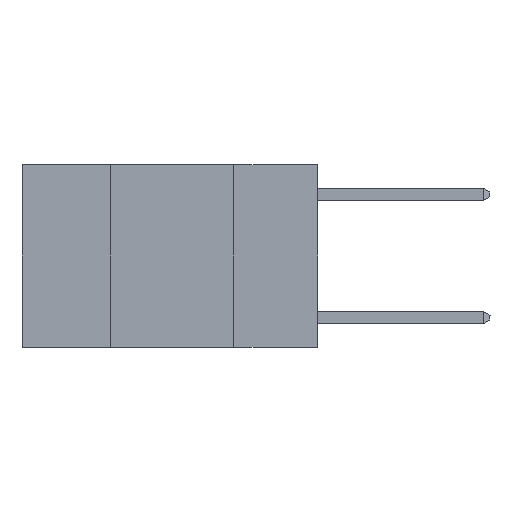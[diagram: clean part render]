
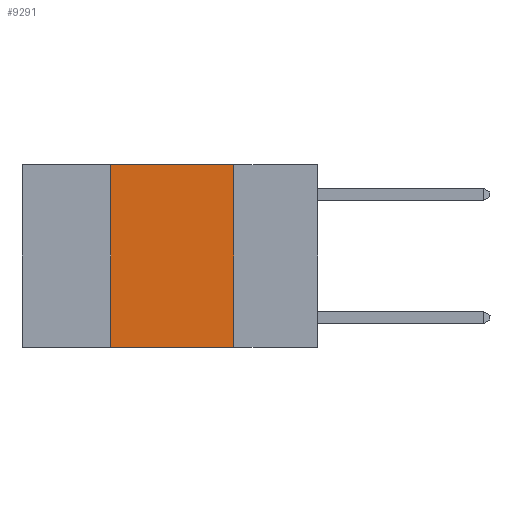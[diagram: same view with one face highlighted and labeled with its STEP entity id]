
A CAD part, left-side view. The second image highlights one B-rep face of the part: STEP entity #9291.
In plain terms, the highlighted planar face has unit normal (-1, 0, 0).
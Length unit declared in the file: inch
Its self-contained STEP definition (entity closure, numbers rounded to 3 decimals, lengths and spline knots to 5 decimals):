
#152 = EDGE_CURVE ( 'NONE', #15434, #3677, #10965, .T. ) ;
#878 = CARTESIAN_POINT ( 'NONE',  ( 0., 0.17, -0.37 ) ) ;
#952 = DIRECTION ( 'NONE',  ( 0., 0., 1. ) ) ;
#1786 = VERTEX_POINT ( 'NONE', #878 ) ;
#1881 = ORIENTED_EDGE ( 'NONE', *, *, #3883, .F. ) ;
#2121 = CARTESIAN_POINT ( 'NONE',  ( 0., 0.42, 0. ) ) ;
#2293 = LINE ( 'NONE', #8303, #11651 ) ;
#2453 = CARTESIAN_POINT ( 'NONE',  ( 0., 0.17, 0. ) ) ;
#2955 = PLANE ( 'NONE',  #13472 ) ;
#3048 = EDGE_CURVE ( 'NONE', #9590, #15434, #2293, .T. ) ;
#3677 = VERTEX_POINT ( 'NONE', #15465 ) ;
#3883 = EDGE_CURVE ( 'NONE', #3677, #1786, #9925, .T. ) ;
#4210 = DIRECTION ( 'NONE',  ( 0., 0., -1. ) ) ;
#4940 = LINE ( 'NONE', #14608, #14290 ) ;
#5136 = ORIENTED_EDGE ( 'NONE', *, *, #152, .F. ) ;
#6676 = VECTOR ( 'NONE', #14672, 39.37008 ) ;
#7719 = EDGE_LOOP ( 'NONE', ( #1881, #5136, #11629, #8777 ) ) ;
#7736 = VECTOR ( 'NONE', #9434, 39.37008 ) ;
#8303 = CARTESIAN_POINT ( 'NONE',  ( 0., 0.42, 0. ) ) ;
#8777 = ORIENTED_EDGE ( 'NONE', *, *, #15588, .T. ) ;
#8819 = CARTESIAN_POINT ( 'NONE',  ( 0., 0.6, 0. ) ) ;
#9291 = ADVANCED_FACE ( 'NONE', ( #14424 ), #2955, .F. ) ;
#9434 = DIRECTION ( 'NONE',  ( 0., -1., 0. ) ) ;
#9590 = VERTEX_POINT ( 'NONE', #15664 ) ;
#9925 = LINE ( 'NONE', #2453, #6676 ) ;
#10965 = LINE ( 'NONE', #8819, #7736 ) ;
#11386 = CARTESIAN_POINT ( 'NONE',  ( 0., 0.6, 0. ) ) ;
#11491 = DIRECTION ( 'NONE',  ( 1., 0., 0. ) ) ;
#11629 = ORIENTED_EDGE ( 'NONE', *, *, #3048, .F. ) ;
#11651 = VECTOR ( 'NONE', #952, 39.37008 ) ;
#13472 = AXIS2_PLACEMENT_3D ( 'NONE', #11386, #11491, #4210 ) ;
#14290 = VECTOR ( 'NONE', #15807, 39.37008 ) ;
#14424 = FACE_OUTER_BOUND ( 'NONE', #7719, .T. ) ;
#14608 = CARTESIAN_POINT ( 'NONE',  ( 0., 0.6, -0.37 ) ) ;
#14672 = DIRECTION ( 'NONE',  ( 0., 0., -1. ) ) ;
#15434 = VERTEX_POINT ( 'NONE', #2121 ) ;
#15465 = CARTESIAN_POINT ( 'NONE',  ( 0., 0.17, 0. ) ) ;
#15588 = EDGE_CURVE ( 'NONE', #9590, #1786, #4940, .T. ) ;
#15664 = CARTESIAN_POINT ( 'NONE',  ( 0., 0.42, -0.37 ) ) ;
#15807 = DIRECTION ( 'NONE',  ( 0., -1., 0. ) ) ;
